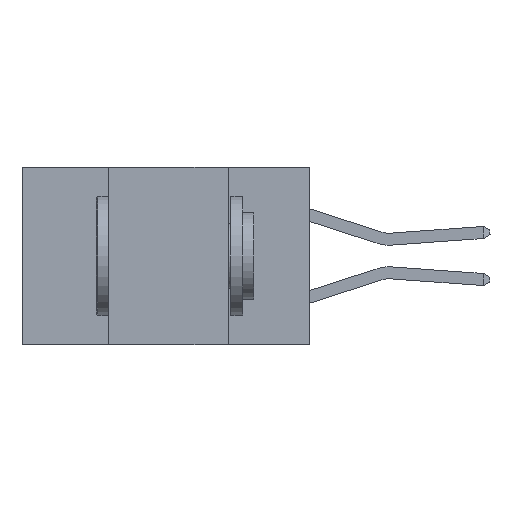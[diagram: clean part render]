
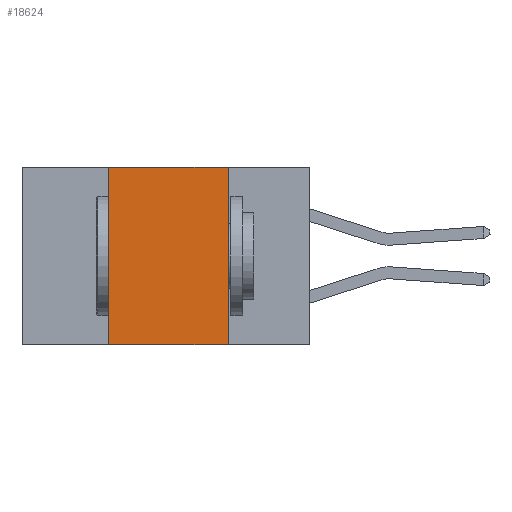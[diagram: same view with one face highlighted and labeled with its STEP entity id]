
A CAD part, left-side view. The second image highlights one B-rep face of the part: STEP entity #18624.
In plain terms, the highlighted planar face has unit normal (-1, 0, 0).
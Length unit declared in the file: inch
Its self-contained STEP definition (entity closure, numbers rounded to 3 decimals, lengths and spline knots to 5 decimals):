
#348 = CARTESIAN_POINT ( 'NONE',  ( 0., 0.42, 0. ) ) ;
#387 = VECTOR ( 'NONE', #19478, 39.37008 ) ;
#397 = ORIENTED_EDGE ( 'NONE', *, *, #12729, .T. ) ;
#792 = LINE ( 'NONE', #17745, #19387 ) ;
#1106 = CARTESIAN_POINT ( 'NONE',  ( 0., 0.6, 0. ) ) ;
#1483 = DIRECTION ( 'NONE',  ( 0., 0., 1. ) ) ;
#1912 = LINE ( 'NONE', #11841, #17574 ) ;
#4123 = ORIENTED_EDGE ( 'NONE', *, *, #7186, .F. ) ;
#6945 = VERTEX_POINT ( 'NONE', #23051 ) ;
#7186 = EDGE_CURVE ( 'NONE', #6945, #19167, #792, .T. ) ;
#7463 = PLANE ( 'NONE',  #15693 ) ;
#7867 = EDGE_CURVE ( 'NONE', #23590, #6945, #25201, .T. ) ;
#9322 = CARTESIAN_POINT ( 'NONE',  ( 0., 0.6, 0. ) ) ;
#9407 = VERTEX_POINT ( 'NONE', #16184 ) ;
#11331 = CARTESIAN_POINT ( 'NONE',  ( 0., 0.17, -0.37 ) ) ;
#11492 = DIRECTION ( 'NONE',  ( 0., -1., 0. ) ) ;
#11841 = CARTESIAN_POINT ( 'NONE',  ( 0., 0.42, 0. ) ) ;
#12729 = EDGE_CURVE ( 'NONE', #9407, #19167, #13422, .T. ) ;
#13422 = LINE ( 'NONE', #19224, #387 ) ;
#14025 = EDGE_CURVE ( 'NONE', #9407, #23590, #1912, .T. ) ;
#15509 = DIRECTION ( 'NONE',  ( 0., 0., -1. ) ) ;
#15693 = AXIS2_PLACEMENT_3D ( 'NONE', #1106, #24394, #24215 ) ;
#16184 = CARTESIAN_POINT ( 'NONE',  ( 0., 0.42, -0.37 ) ) ;
#16366 = FACE_OUTER_BOUND ( 'NONE', #22961, .T. ) ;
#16749 = VECTOR ( 'NONE', #11492, 39.37008 ) ;
#17574 = VECTOR ( 'NONE', #1483, 39.37008 ) ;
#17745 = CARTESIAN_POINT ( 'NONE',  ( 0., 0.17, 0. ) ) ;
#18624 = ADVANCED_FACE ( 'NONE', ( #16366 ), #7463, .F. ) ;
#19167 = VERTEX_POINT ( 'NONE', #11331 ) ;
#19224 = CARTESIAN_POINT ( 'NONE',  ( 0., 0.6, -0.37 ) ) ;
#19387 = VECTOR ( 'NONE', #15509, 39.37008 ) ;
#19478 = DIRECTION ( 'NONE',  ( 0., -1., 0. ) ) ;
#20502 = ORIENTED_EDGE ( 'NONE', *, *, #7867, .F. ) ;
#22961 = EDGE_LOOP ( 'NONE', ( #4123, #20502, #25402, #397 ) ) ;
#23051 = CARTESIAN_POINT ( 'NONE',  ( 0., 0.17, 0. ) ) ;
#23590 = VERTEX_POINT ( 'NONE', #348 ) ;
#24215 = DIRECTION ( 'NONE',  ( 0., 0., -1. ) ) ;
#24394 = DIRECTION ( 'NONE',  ( 1., 0., 0. ) ) ;
#25201 = LINE ( 'NONE', #9322, #16749 ) ;
#25402 = ORIENTED_EDGE ( 'NONE', *, *, #14025, .F. ) ;
